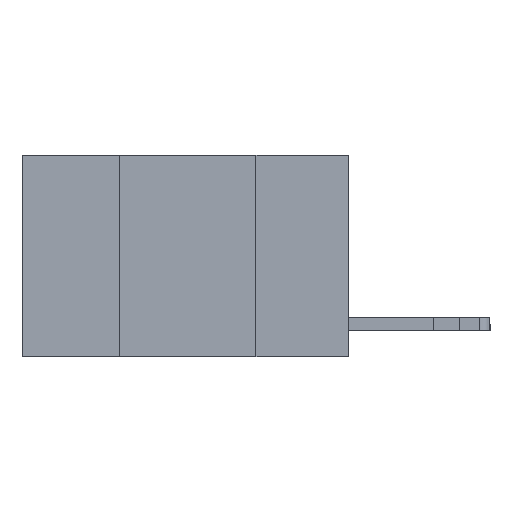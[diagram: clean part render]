
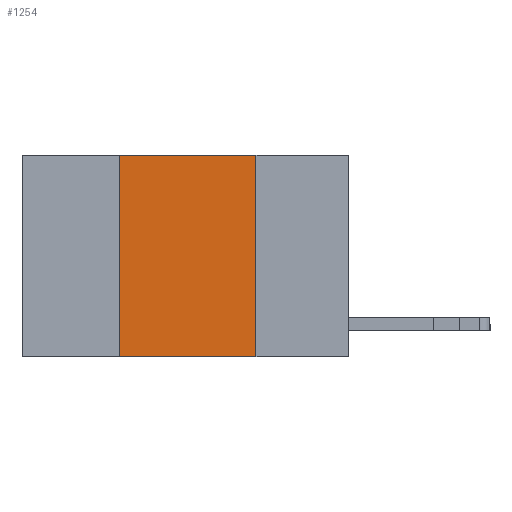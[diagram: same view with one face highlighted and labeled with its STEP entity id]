
A CAD part, left-side view. The second image highlights one B-rep face of the part: STEP entity #1254.
In plain terms, the highlighted planar face has unit normal (-1, 0, 0).
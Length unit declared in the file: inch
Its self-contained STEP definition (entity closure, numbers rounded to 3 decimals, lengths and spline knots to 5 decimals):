
#237 = VERTEX_POINT ( 'NONE', #11789 ) ;
#328 = DIRECTION ( 'NONE',  ( 0., 0., -1. ) ) ;
#746 = CARTESIAN_POINT ( 'NONE',  ( 0., 0.17, -0.37 ) ) ;
#931 = ORIENTED_EDGE ( 'NONE', *, *, #9723, .F. ) ;
#1254 = ADVANCED_FACE ( 'NONE', ( #9828 ), #14493, .F. ) ;
#2499 = ORIENTED_EDGE ( 'NONE', *, *, #5338, .F. ) ;
#2728 = CARTESIAN_POINT ( 'NONE',  ( 0., 0.17, 0. ) ) ;
#3058 = EDGE_CURVE ( 'NONE', #13755, #5525, #13508, .T. ) ;
#3348 = DIRECTION ( 'NONE',  ( 1., 0., 0. ) ) ;
#3663 = CARTESIAN_POINT ( 'NONE',  ( 0., 0.42, -0.37 ) ) ;
#4125 = VECTOR ( 'NONE', #328, 39.37008 ) ;
#4419 = CARTESIAN_POINT ( 'NONE',  ( 0., 0.6, 0. ) ) ;
#4460 = EDGE_LOOP ( 'NONE', ( #2499, #931, #10422, #9525 ) ) ;
#4616 = VECTOR ( 'NONE', #5716, 39.37008 ) ;
#5338 = EDGE_CURVE ( 'NONE', #6140, #5525, #12047, .T. ) ;
#5525 = VERTEX_POINT ( 'NONE', #746 ) ;
#5716 = DIRECTION ( 'NONE',  ( 0., 0., 1. ) ) ;
#5885 = LINE ( 'NONE', #11151, #4616 ) ;
#6140 = VERTEX_POINT ( 'NONE', #14226 ) ;
#8276 = EDGE_CURVE ( 'NONE', #13755, #237, #5885, .T. ) ;
#8544 = DIRECTION ( 'NONE',  ( 0., 0., -1. ) ) ;
#9488 = DIRECTION ( 'NONE',  ( 0., -1., 0. ) ) ;
#9525 = ORIENTED_EDGE ( 'NONE', *, *, #3058, .T. ) ;
#9561 = VECTOR ( 'NONE', #12358, 39.37008 ) ;
#9723 = EDGE_CURVE ( 'NONE', #237, #6140, #10823, .T. ) ;
#9828 = FACE_OUTER_BOUND ( 'NONE', #4460, .T. ) ;
#10422 = ORIENTED_EDGE ( 'NONE', *, *, #8276, .F. ) ;
#10823 = LINE ( 'NONE', #4419, #9561 ) ;
#11151 = CARTESIAN_POINT ( 'NONE',  ( 0., 0.42, 0. ) ) ;
#11187 = CARTESIAN_POINT ( 'NONE',  ( 0., 0.6, -0.37 ) ) ;
#11789 = CARTESIAN_POINT ( 'NONE',  ( 0., 0.42, 0. ) ) ;
#12047 = LINE ( 'NONE', #2728, #4125 ) ;
#12170 = AXIS2_PLACEMENT_3D ( 'NONE', #13689, #3348, #8544 ) ;
#12358 = DIRECTION ( 'NONE',  ( 0., -1., 0. ) ) ;
#13508 = LINE ( 'NONE', #11187, #14661 ) ;
#13689 = CARTESIAN_POINT ( 'NONE',  ( 0., 0.6, 0. ) ) ;
#13755 = VERTEX_POINT ( 'NONE', #3663 ) ;
#14226 = CARTESIAN_POINT ( 'NONE',  ( 0., 0.17, 0. ) ) ;
#14493 = PLANE ( 'NONE',  #12170 ) ;
#14661 = VECTOR ( 'NONE', #9488, 39.37008 ) ;
